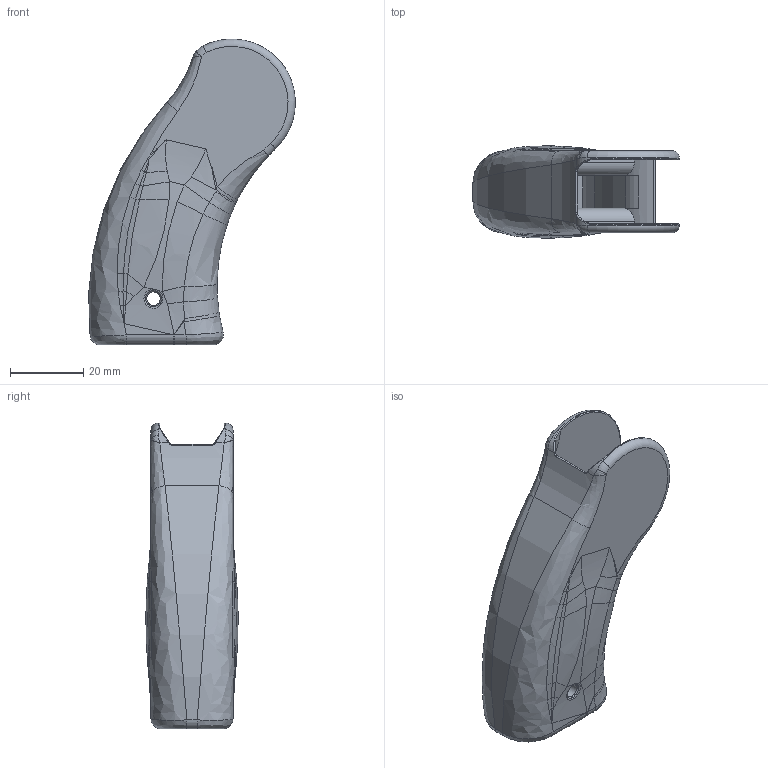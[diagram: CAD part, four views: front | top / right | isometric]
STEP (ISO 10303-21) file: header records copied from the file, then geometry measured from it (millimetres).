
FILE_DESCRIPTION(/* description */ (''),/* implementation_level */ '2;1');
FILE_NAME(/* name */ 'BG Standard.step',/* time_stamp */ '2021-08-04T10:29:18-04:00',/* author */ (''),/* organization */ (''),/* preprocessor_version */ 'ST-DEVELOPER v18.1',/* originating_system */ 'Autodesk Translation Framework v10.9.0.1377',/* authorisation */ '');
FILE_SCHEMA (('AUTOMOTIVE_DESIGN { 1 0 10303 214 3 1 1 }'));
Length unit declared in the file: millimetre
Products named in the file (1): BG Standard
Bounding box: 56.4 x 25.2 x 83.48 mm (x, y, z)
Volume: 35303.9 mm3; surface area: 15304.8 mm2
Topology: 1 solids, 1 shells, 198 faces, 495 edges, 286 vertices
Faces by surface type: bspline 116, cylinder 43, torus 20, plane 19
Full cylindrical faces by diameter (mm): 3.71 x2
Entity records: 9745 total; most frequent: CARTESIAN_POINT 5796, ORIENTED_EDGE 958, DIRECTION 579, EDGE_CURVE 479, VERTEX_POINT 286, AXIS2_PLACEMENT_3D 257, B_SPLINE_CURVE_WITH_KNOTS 240, EDGE_LOOP 205
